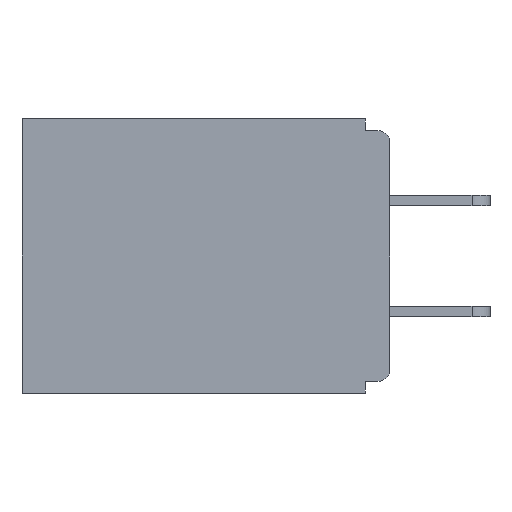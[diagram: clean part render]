
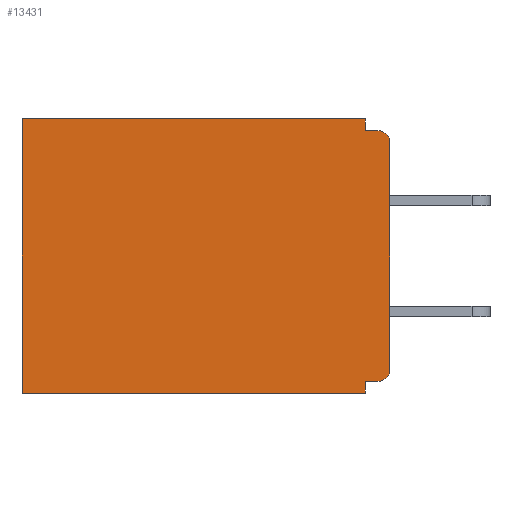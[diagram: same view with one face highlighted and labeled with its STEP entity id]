
A CAD part, left-side view. The second image highlights one B-rep face of the part: STEP entity #13431.
In plain terms, the highlighted planar face has unit normal (-1, 0, 0).
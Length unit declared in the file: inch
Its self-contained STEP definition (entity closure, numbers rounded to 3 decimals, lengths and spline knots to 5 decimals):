
#521 = EDGE_CURVE ( 'NONE', #6508, #1587, #18780, .T. ) ;
#616 = VERTEX_POINT ( 'NONE', #884 ) ;
#705 = VERTEX_POINT ( 'NONE', #17407 ) ;
#781 = ORIENTED_EDGE ( 'NONE', *, *, #17018, .F. ) ;
#884 = CARTESIAN_POINT ( 'NONE',  ( 0.298, 0.031, -0.015 ) ) ;
#1110 = CARTESIAN_POINT ( 'NONE',  ( 0.298, 0.031, -0.343 ) ) ;
#1587 = VERTEX_POINT ( 'NONE', #7214 ) ;
#1715 = VERTEX_POINT ( 'NONE', #4168 ) ;
#1885 = CARTESIAN_POINT ( 'NONE',  ( 0.298, 0., -0.343 ) ) ;
#1964 = ORIENTED_EDGE ( 'NONE', *, *, #521, .F. ) ;
#2366 = EDGE_CURVE ( 'NONE', #705, #6508, #9798, .T. ) ;
#2650 = LINE ( 'NONE', #5158, #14887 ) ;
#2888 = CARTESIAN_POINT ( 'NONE',  ( 0.298, 0., 0. ) ) ;
#3000 = PLANE ( 'NONE',  #5541 ) ;
#3398 = DIRECTION ( 'NONE',  ( 0., 0., -1. ) ) ;
#3495 = CARTESIAN_POINT ( 'NONE',  ( 0.298, 0.46, -0.343 ) ) ;
#3840 = CARTESIAN_POINT ( 'NONE',  ( 0.298, 0., -0.313 ) ) ;
#4168 = CARTESIAN_POINT ( 'NONE',  ( 0.298, 0.015, -0.015 ) ) ;
#4234 = VECTOR ( 'NONE', #17240, 39.37008 ) ;
#4520 = EDGE_CURVE ( 'NONE', #10762, #1715, #17496, .T. ) ;
#4534 = LINE ( 'NONE', #1885, #10095 ) ;
#4725 = ORIENTED_EDGE ( 'NONE', *, *, #9465, .T. ) ;
#5090 = EDGE_CURVE ( 'NONE', #14616, #616, #14213, .T. ) ;
#5158 = CARTESIAN_POINT ( 'NONE',  ( 0.298, 0., 0. ) ) ;
#5258 = VECTOR ( 'NONE', #14609, 39.37008 ) ;
#5343 = AXIS2_PLACEMENT_3D ( 'NONE', #6441, #16756, #7953 ) ;
#5429 = ORIENTED_EDGE ( 'NONE', *, *, #4520, .T. ) ;
#5537 = ORIENTED_EDGE ( 'NONE', *, *, #10334, .T. ) ;
#5541 = AXIS2_PLACEMENT_3D ( 'NONE', #13295, #10377, #7328 ) ;
#5563 = ORIENTED_EDGE ( 'NONE', *, *, #11025, .F. ) ;
#6441 = CARTESIAN_POINT ( 'NONE',  ( 0.298, 0.015, -0.03 ) ) ;
#6508 = VERTEX_POINT ( 'NONE', #10133 ) ;
#7043 = VERTEX_POINT ( 'NONE', #3495 ) ;
#7214 = CARTESIAN_POINT ( 'NONE',  ( 0.298, 0.031, -0.343 ) ) ;
#7328 = DIRECTION ( 'NONE',  ( 0., 0., -1. ) ) ;
#7659 = CARTESIAN_POINT ( 'NONE',  ( 0.298, 0.015, -0.313 ) ) ;
#7764 = LINE ( 'NONE', #12426, #12561 ) ;
#7953 = DIRECTION ( 'NONE',  ( 0., 0., -1. ) ) ;
#8106 = EDGE_CURVE ( 'NONE', #705, #8446, #15237, .T. ) ;
#8446 = VERTEX_POINT ( 'NONE', #3840 ) ;
#9326 = VECTOR ( 'NONE', #16063, 39.37008 ) ;
#9465 = EDGE_CURVE ( 'NONE', #10292, #7043, #16850, .T. ) ;
#9798 = LINE ( 'NONE', #13356, #9326 ) ;
#10095 = VECTOR ( 'NONE', #15733, 39.37008 ) ;
#10133 = CARTESIAN_POINT ( 'NONE',  ( 0.298, 0.031, -0.328 ) ) ;
#10273 = CARTESIAN_POINT ( 'NONE',  ( 0.298, 0.46, 0. ) ) ;
#10292 = VERTEX_POINT ( 'NONE', #10273 ) ;
#10334 = EDGE_CURVE ( 'NONE', #14616, #10292, #16550, .T. ) ;
#10377 = DIRECTION ( 'NONE',  ( 1., 0., 0. ) ) ;
#10443 = DIRECTION ( 'NONE',  ( 0., 0., -1. ) ) ;
#10762 = VERTEX_POINT ( 'NONE', #13057 ) ;
#10833 = CARTESIAN_POINT ( 'NONE',  ( 0.298, 0.46, 0. ) ) ;
#11025 = EDGE_CURVE ( 'NONE', #1587, #7043, #4534, .T. ) ;
#11246 = DIRECTION ( 'NONE',  ( 0., -1., 0. ) ) ;
#11251 = VECTOR ( 'NONE', #16653, 39.37008 ) ;
#12426 = CARTESIAN_POINT ( 'NONE',  ( 0.298, 0., -0.015 ) ) ;
#12561 = VECTOR ( 'NONE', #11246, 39.37008 ) ;
#13041 = EDGE_LOOP ( 'NONE', ( #5429, #781, #14579, #5537, #4725, #5563, #1964, #17967, #17686, #14474 ) ) ;
#13057 = CARTESIAN_POINT ( 'NONE',  ( 0.298, 0., -0.03 ) ) ;
#13295 = CARTESIAN_POINT ( 'NONE',  ( 0.298, 0., 0. ) ) ;
#13356 = CARTESIAN_POINT ( 'NONE',  ( 0.298, 0., -0.328 ) ) ;
#13431 = ADVANCED_FACE ( 'NONE', ( #18912 ), #3000, .F. ) ;
#14213 = LINE ( 'NONE', #1110, #5258 ) ;
#14246 = CARTESIAN_POINT ( 'NONE',  ( 0.298, 0.031, -0.343 ) ) ;
#14474 = ORIENTED_EDGE ( 'NONE', *, *, #16743, .F. ) ;
#14579 = ORIENTED_EDGE ( 'NONE', *, *, #5090, .F. ) ;
#14609 = DIRECTION ( 'NONE',  ( 0., 0., -1. ) ) ;
#14616 = VERTEX_POINT ( 'NONE', #14689 ) ;
#14689 = CARTESIAN_POINT ( 'NONE',  ( 0.298, 0.031, 0. ) ) ;
#14887 = VECTOR ( 'NONE', #16750, 39.37008 ) ;
#15237 = CIRCLE ( 'NONE', #16736, 0.015 ) ;
#15733 = DIRECTION ( 'NONE',  ( 0., 1., 0. ) ) ;
#16063 = DIRECTION ( 'NONE',  ( 0., 1., 0. ) ) ;
#16550 = LINE ( 'NONE', #2888, #11251 ) ;
#16588 = DIRECTION ( 'NONE',  ( -1., 0., 0. ) ) ;
#16653 = DIRECTION ( 'NONE',  ( 0., 1., 0. ) ) ;
#16736 = AXIS2_PLACEMENT_3D ( 'NONE', #7659, #16588, #10443 ) ;
#16743 = EDGE_CURVE ( 'NONE', #10762, #8446, #2650, .T. ) ;
#16750 = DIRECTION ( 'NONE',  ( 0., 0., -1. ) ) ;
#16756 = DIRECTION ( 'NONE',  ( -1., 0., 0. ) ) ;
#16850 = LINE ( 'NONE', #10833, #17073 ) ;
#17018 = EDGE_CURVE ( 'NONE', #616, #1715, #7764, .T. ) ;
#17073 = VECTOR ( 'NONE', #3398, 39.37008 ) ;
#17240 = DIRECTION ( 'NONE',  ( 0., 0., -1. ) ) ;
#17407 = CARTESIAN_POINT ( 'NONE',  ( 0.298, 0.015, -0.328 ) ) ;
#17496 = CIRCLE ( 'NONE', #5343, 0.015 ) ;
#17686 = ORIENTED_EDGE ( 'NONE', *, *, #8106, .T. ) ;
#17967 = ORIENTED_EDGE ( 'NONE', *, *, #2366, .F. ) ;
#18780 = LINE ( 'NONE', #14246, #4234 ) ;
#18912 = FACE_OUTER_BOUND ( 'NONE', #13041, .T. ) ;
